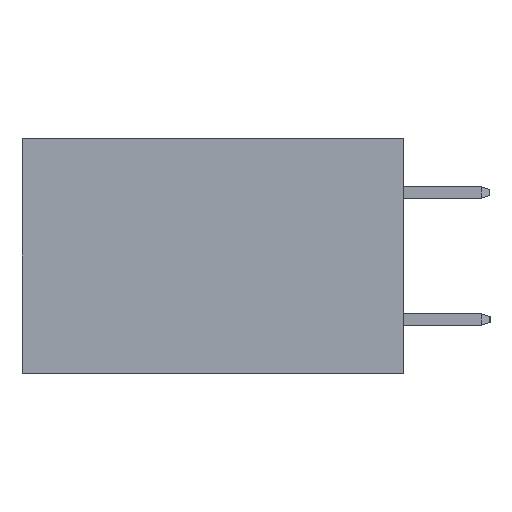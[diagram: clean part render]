
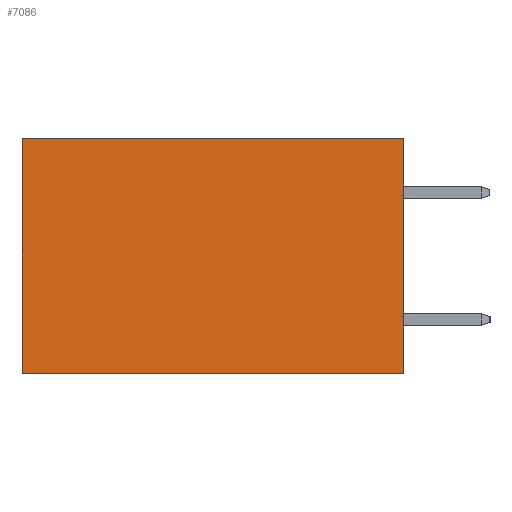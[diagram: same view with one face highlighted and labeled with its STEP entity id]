
A CAD part, left-side view. The second image highlights one B-rep face of the part: STEP entity #7086.
In plain terms, the highlighted planar face has unit normal (-1, 0, 0).
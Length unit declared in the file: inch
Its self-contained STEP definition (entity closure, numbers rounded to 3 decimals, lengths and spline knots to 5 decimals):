
#108 = VECTOR ( 'NONE', #4775, 39.37008 ) ;
#415 = EDGE_CURVE ( 'NONE', #7303, #9379, #3659, .T. ) ;
#1096 = LINE ( 'NONE', #5979, #108 ) ;
#1631 = FACE_OUTER_BOUND ( 'NONE', #2887, .T. ) ;
#2447 = DIRECTION ( 'NONE',  ( 0., 1., 0. ) ) ;
#2887 = EDGE_LOOP ( 'NONE', ( #3024, #14837, #4185, #8943 ) ) ;
#3024 = ORIENTED_EDGE ( 'NONE', *, *, #9062, .T. ) ;
#3070 = DIRECTION ( 'NONE',  ( 1., 0., 0. ) ) ;
#3367 = EDGE_CURVE ( 'NONE', #14173, #13091, #14514, .T. ) ;
#3560 = AXIS2_PLACEMENT_3D ( 'NONE', #11289, #3070, #10221 ) ;
#3659 = LINE ( 'NONE', #13471, #10162 ) ;
#4185 = ORIENTED_EDGE ( 'NONE', *, *, #14721, .F. ) ;
#4426 = CARTESIAN_POINT ( 'NONE',  ( 0.2875, 0., -0.37 ) ) ;
#4775 = DIRECTION ( 'NONE',  ( 0., 0., -1. ) ) ;
#5051 = VECTOR ( 'NONE', #10656, 39.37008 ) ;
#5979 = CARTESIAN_POINT ( 'NONE',  ( 0.2875, 0., 0. ) ) ;
#6016 = CARTESIAN_POINT ( 'NONE',  ( 0.2875, 0.6, 0. ) ) ;
#6318 = CARTESIAN_POINT ( 'NONE',  ( 0.2875, 0.6, 0. ) ) ;
#7086 = ADVANCED_FACE ( 'NONE', ( #1631 ), #12724, .F. ) ;
#7234 = LINE ( 'NONE', #6016, #10531 ) ;
#7303 = VERTEX_POINT ( 'NONE', #4426 ) ;
#8407 = CARTESIAN_POINT ( 'NONE',  ( 0.2875, 0., 0. ) ) ;
#8943 = ORIENTED_EDGE ( 'NONE', *, *, #3367, .T. ) ;
#9062 = EDGE_CURVE ( 'NONE', #13091, #9379, #7234, .T. ) ;
#9379 = VERTEX_POINT ( 'NONE', #13977 ) ;
#10162 = VECTOR ( 'NONE', #2447, 39.37008 ) ;
#10221 = DIRECTION ( 'NONE',  ( 0., 0., -1. ) ) ;
#10531 = VECTOR ( 'NONE', #10695, 39.37008 ) ;
#10656 = DIRECTION ( 'NONE',  ( 0., 1., 0. ) ) ;
#10695 = DIRECTION ( 'NONE',  ( 0., 0., -1. ) ) ;
#11289 = CARTESIAN_POINT ( 'NONE',  ( 0.2875, 0., 0. ) ) ;
#12724 = PLANE ( 'NONE',  #3560 ) ;
#13091 = VERTEX_POINT ( 'NONE', #6318 ) ;
#13471 = CARTESIAN_POINT ( 'NONE',  ( 0.2875, 0., -0.37 ) ) ;
#13977 = CARTESIAN_POINT ( 'NONE',  ( 0.2875, 0.6, -0.37 ) ) ;
#14173 = VERTEX_POINT ( 'NONE', #15684 ) ;
#14514 = LINE ( 'NONE', #8407, #5051 ) ;
#14721 = EDGE_CURVE ( 'NONE', #14173, #7303, #1096, .T. ) ;
#14837 = ORIENTED_EDGE ( 'NONE', *, *, #415, .F. ) ;
#15684 = CARTESIAN_POINT ( 'NONE',  ( 0.2875, 0., 0. ) ) ;
